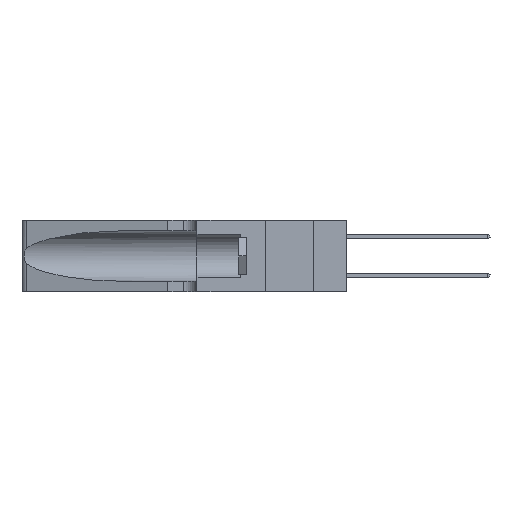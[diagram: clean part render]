
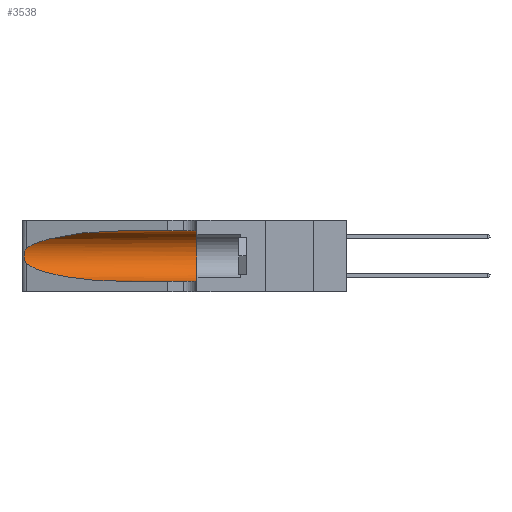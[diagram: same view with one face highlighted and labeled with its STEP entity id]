
A CAD part, left-side view. The second image highlights one B-rep face of the part: STEP entity #3538.
In plain terms, the highlighted cylindrical face has radius 3.308 mm (diameter 6.617 mm), a partial arc.
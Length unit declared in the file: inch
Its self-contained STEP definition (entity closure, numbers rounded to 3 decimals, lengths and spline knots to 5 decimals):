
#1253 = CARTESIAN_POINT ( 'NONE',  ( 0.2373, 1.15595, 0.08982 ) ) ;
#1769 = CARTESIAN_POINT ( 'NONE',  ( 0.1305, 0.72297, 0.31525 ) ) ;
#2872 = CARTESIAN_POINT ( 'NONE',  ( 0.25787, 1.23484, 0.2124 ) ) ;
#2962 = CARTESIAN_POINT ( 'NONE',  ( 0.25639, 1.23184, 0.21858 ) ) ;
#3538 = ADVANCED_FACE ( 'NONE', ( #17519 ), #18613, .F. ) ;
#4828 = EDGE_CURVE ( 'NONE', #25897, #44209, #12620, .T. ) ;
#5197 = CARTESIAN_POINT ( 'NONE',  ( 0.18966, 0.96281, 0.05475 ) ) ;
#5886 = CARTESIAN_POINT ( 'NONE',  ( 0.1305, 0.72297, 0.05475 ) ) ;
#6326 = CARTESIAN_POINT ( 'NONE',  ( 0.25854, 1.2359, 0.20912 ) ) ;
#6483 = ORIENTED_EDGE ( 'NONE', *, *, #27769, .F. ) ;
#6740 = CARTESIAN_POINT ( 'NONE',  ( 0.1305, 1.61858, 0.185 ) ) ;
#8224 = EDGE_LOOP ( 'NONE', ( #11696, #15568, #30602, #9752, #19202, #6483 ) ) ;
#8626 = EDGE_CURVE ( 'NONE', #16371, #25897, #10047, .T. ) ;
#9752 = ORIENTED_EDGE ( 'NONE', *, *, #4828, .T. ) ;
#10047 =( BOUNDED_CURVE ( )  B_SPLINE_CURVE ( 3, ( #18856, #1253, #5197, #28554 ),
 .UNSPECIFIED., .F., .F. ) 
 B_SPLINE_CURVE_WITH_KNOTS ( ( 4, 4 ),
 ( 3.44316, 4.71239 ),
 .UNSPECIFIED. ) 
 CURVE ( )  GEOMETRIC_REPRESENTATION_ITEM ( )  RATIONAL_B_SPLINE_CURVE ( ( 1., 0.87, 0.87, 1. ) ) 
 REPRESENTATION_ITEM ( '' )  );
#10316 = CARTESIAN_POINT ( 'NONE',  ( 0.18966, 0.96281, 0.31525 ) ) ;
#11696 = ORIENTED_EDGE ( 'NONE', *, *, #16825, .T. ) ;
#11953 = DIRECTION ( 'NONE',  ( 0., -1., 0. ) ) ;
#12620 = LINE ( 'NONE', #24050, #38247 ) ;
#13752 = CARTESIAN_POINT ( 'NONE',  ( 0.2373, 1.15595, 0.28018 ) ) ;
#15568 = ORIENTED_EDGE ( 'NONE', *, *, #25978, .T. ) ;
#16371 = VERTEX_POINT ( 'NONE', #33090 ) ;
#16560 = VERTEX_POINT ( 'NONE', #34246 ) ;
#16825 = EDGE_CURVE ( 'NONE', #16560, #28222, #28408, .T. ) ;
#16826 = CARTESIAN_POINT ( 'NONE',  ( 0.26075, 1.23896, 0.178 ) ) ;
#17329 = CARTESIAN_POINT ( 'NONE',  ( 0.1305, 0.35, 0.05475 ) ) ;
#17519 = FACE_OUTER_BOUND ( 'NONE', #8224, .T. ) ;
#18613 = CYLINDRICAL_SURFACE ( 'NONE', #34776, 0.13025 ) ;
#18856 = CARTESIAN_POINT ( 'NONE',  ( 0.25487, 1.22718, 0.14631 ) ) ;
#19202 = ORIENTED_EDGE ( 'NONE', *, *, #23260, .F. ) ;
#20422 = CARTESIAN_POINT ( 'NONE',  ( 0.25555, 1.22994, 0.2215 ) ) ;
#20583 = CARTESIAN_POINT ( 'NONE',  ( 0.25487, 1.22718, 0.22369 ) ) ;
#20721 = CARTESIAN_POINT ( 'NONE',  ( 0.25639, 1.23186, 0.15144 ) ) ;
#22612 = CARTESIAN_POINT ( 'NONE',  ( 0.1305, 0.35, 0.185 ) ) ;
#23260 = EDGE_CURVE ( 'NONE', #33153, #44209, #26175, .T. ) ;
#23734 = CARTESIAN_POINT ( 'NONE',  ( 0.25555, 1.22993, 0.14849 ) ) ;
#24011 = CARTESIAN_POINT ( 'NONE',  ( 0.25487, 1.22718, 0.14631 ) ) ;
#24050 = CARTESIAN_POINT ( 'NONE',  ( 0.1305, 1.61858, 0.05475 ) ) ;
#24276 = DIRECTION ( 'NONE',  ( 0., 0., -1. ) ) ;
#25897 = VERTEX_POINT ( 'NONE', #5886 ) ;
#25978 = EDGE_CURVE ( 'NONE', #28222, #16371, #26545, .T. ) ;
#26175 = CIRCLE ( 'NONE', #43256, 0.13025 ) ;
#26545 = B_SPLINE_CURVE_WITH_KNOTS ( 'NONE', 3,
 ( #20583, #20422, #2962, #2872, #6326, #30697, #33978, #16826, #44065, #30256, #40868, #20721, #23734, #24011 ),
 .UNSPECIFIED., .F., .F.,
 ( 4, 2, 2, 2, 2, 2, 4 ),
 ( 0., 0.00027, 0.00053, 0.00107, 0.0016, 0.00187, 0.00214 ),
 .UNSPECIFIED. ) ;
#27769 = EDGE_CURVE ( 'NONE', #16560, #33153, #30420, .T. ) ;
#27791 = CARTESIAN_POINT ( 'NONE',  ( 0.25487, 1.22718, 0.22369 ) ) ;
#28222 = VERTEX_POINT ( 'NONE', #36798 ) ;
#28408 =( BOUNDED_CURVE ( )  B_SPLINE_CURVE ( 3, ( #1769, #10316, #13752, #27791 ),
 .UNSPECIFIED., .F., .F. ) 
 B_SPLINE_CURVE_WITH_KNOTS ( ( 4, 4 ),
 ( 1.5708, 2.84003 ),
 .UNSPECIFIED. ) 
 CURVE ( )  GEOMETRIC_REPRESENTATION_ITEM ( )  RATIONAL_B_SPLINE_CURVE ( ( 1., 0.87, 0.87, 1. ) ) 
 REPRESENTATION_ITEM ( '' )  );
#28554 = CARTESIAN_POINT ( 'NONE',  ( 0.1305, 0.72297, 0.05475 ) ) ;
#29536 = DIRECTION ( 'NONE',  ( 0., -1., 0. ) ) ;
#30256 = CARTESIAN_POINT ( 'NONE',  ( 0.25856, 1.23593, 0.16098 ) ) ;
#30420 = LINE ( 'NONE', #33255, #41102 ) ;
#30602 = ORIENTED_EDGE ( 'NONE', *, *, #8626, .T. ) ;
#30697 = CARTESIAN_POINT ( 'NONE',  ( 0.26018, 1.23835, 0.19895 ) ) ;
#33090 = CARTESIAN_POINT ( 'NONE',  ( 0.25487, 1.22718, 0.14631 ) ) ;
#33153 = VERTEX_POINT ( 'NONE', #43742 ) ;
#33255 = CARTESIAN_POINT ( 'NONE',  ( 0.1305, 1.61858, 0.31525 ) ) ;
#33978 = CARTESIAN_POINT ( 'NONE',  ( 0.26075, 1.23896, 0.19203 ) ) ;
#34246 = CARTESIAN_POINT ( 'NONE',  ( 0.1305, 0.72297, 0.31525 ) ) ;
#34776 = AXIS2_PLACEMENT_3D ( 'NONE', #6740, #41415, #24276 ) ;
#35334 = DIRECTION ( 'NONE',  ( 0., 0., 1. ) ) ;
#36798 = CARTESIAN_POINT ( 'NONE',  ( 0.25487, 1.22718, 0.22369 ) ) ;
#38006 = DIRECTION ( 'NONE',  ( 0., 1., 0. ) ) ;
#38247 = VECTOR ( 'NONE', #11953, 39.37008 ) ;
#40868 = CARTESIAN_POINT ( 'NONE',  ( 0.25789, 1.23486, 0.15765 ) ) ;
#41102 = VECTOR ( 'NONE', #29536, 39.37008 ) ;
#41415 = DIRECTION ( 'NONE',  ( 0., -1., 0. ) ) ;
#43256 = AXIS2_PLACEMENT_3D ( 'NONE', #22612, #38006, #35334 ) ;
#43742 = CARTESIAN_POINT ( 'NONE',  ( 0.1305, 0.35, 0.31525 ) ) ;
#44065 = CARTESIAN_POINT ( 'NONE',  ( 0.26017, 1.23833, 0.17102 ) ) ;
#44209 = VERTEX_POINT ( 'NONE', #17329 ) ;
